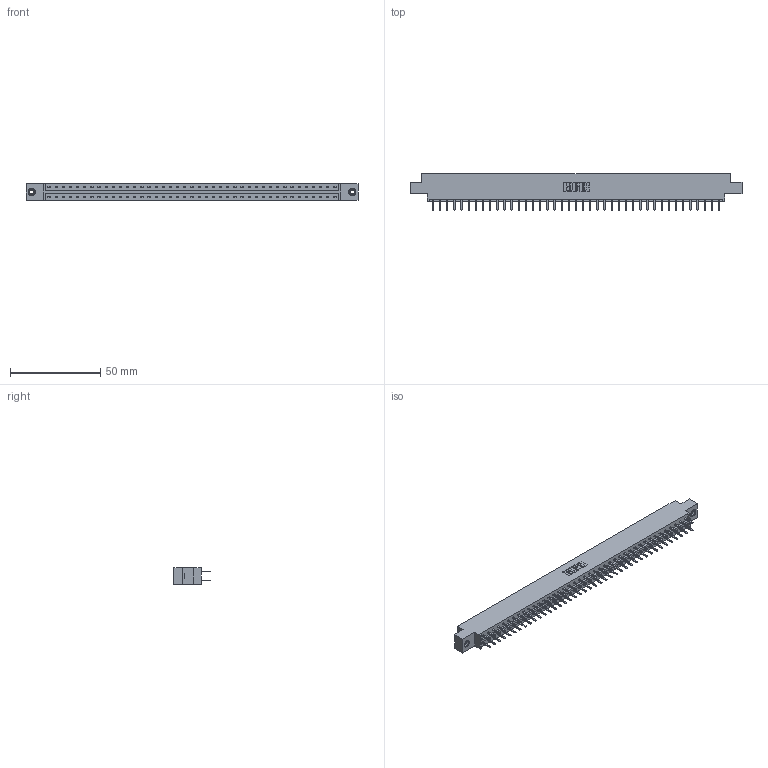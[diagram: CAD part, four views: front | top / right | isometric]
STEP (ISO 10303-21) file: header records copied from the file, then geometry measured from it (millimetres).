
FILE_DESCRIPTION (( 'STEP AP203' ), '1' );
FILE_NAME ('833-082-520-808.STEP', '2020-06-05T23:06:00', ( '' ), ( '' ), 'SwSTEP 2.0', 'SolidWorks 2020', '' );
FILE_SCHEMA (( 'CONFIG_CONTROL_DESIGN' ));
Length unit declared in the file: inch
Products named in the file (4): 345-250-001_345-250-003-102; 345-292-001_345-293-120; 833-082-520-808; 833 Part_Offset - .156 Dia - TI
Assembly tree (85 placements, depth 2):
  833-082-520-808
    833 Part_Offset - .156 Dia - TI
    345-292-001_345-293-120  x82
    345-250-001_345-250-003-102  x2
Bounding box: 184 x 20.02 x 9.4 mm (x, y, z)
Volume: 18505.4 mm3; surface area: 22014.3 mm2
Topology: 85 solids, 85 shells, 4770 faces, 13825 edges, 8990 vertices
Faces by surface type: plane 3222, cylinder 1532, cone 12, torus 4
Entity records: 27938 total; most frequent: CARTESIAN_POINT 4629, ORIENTED_EDGE 4546, DIRECTION 3975, EDGE_CURVE 2273, VECTOR 2121, LINE 2121, VERTEX_POINT 1508, AXIS2_PLACEMENT_3D 927
